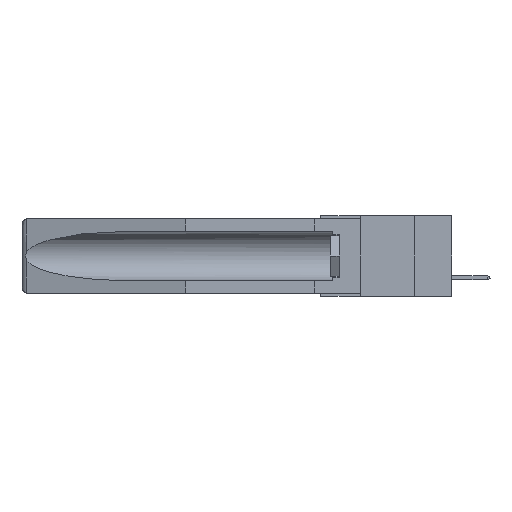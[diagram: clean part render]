
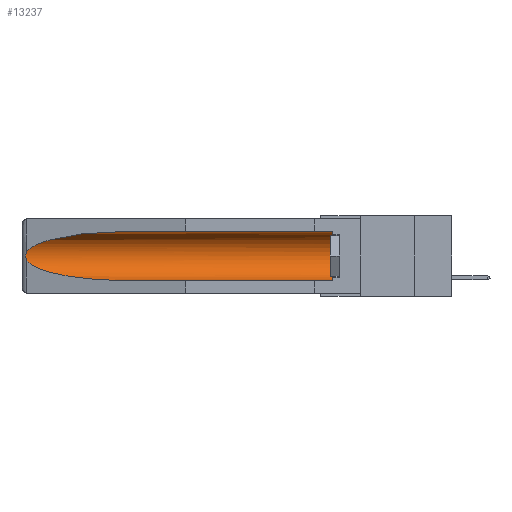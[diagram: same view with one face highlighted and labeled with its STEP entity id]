
A CAD part, left-side view. The second image highlights one B-rep face of the part: STEP entity #13237.
In plain terms, the highlighted cylindrical face has radius 2.857 mm (diameter 5.715 mm), a partial arc.
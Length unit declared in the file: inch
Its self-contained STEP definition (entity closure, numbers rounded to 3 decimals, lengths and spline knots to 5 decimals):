
#164 = CARTESIAN_POINT ( 'NONE',  ( 0.25451, 1.48313, -0.24835 ) ) ;
#382 = CARTESIAN_POINT ( 'NONE',  ( 0.25451, 1.48313, -0.09465 ) ) ;
#494 = CARTESIAN_POINT ( 'NONE',  ( 0.26537, 1.52718, -0.14972 ) ) ;
#1466 = CARTESIAN_POINT ( 'NONE',  ( 0.155, -0.30754, -0.1715 ) ) ;
#1634 = ORIENTED_EDGE ( 'NONE', *, *, #14300, .T. ) ;
#1669 = CARTESIAN_POINT ( 'NONE',  ( 0.2675, 1.53308, -0.16763 ) ) ;
#1854 = CARTESIAN_POINT ( 'NONE',  ( 0.155, -0.30754, -0.059 ) ) ;
#1901 = EDGE_CURVE ( 'NONE', #17333, #27058, #24719, .T. ) ;
#3389 = CARTESIAN_POINT ( 'NONE',  ( 0.155, 0.126, -0.1715 ) ) ;
#4767 = AXIS2_PLACEMENT_3D ( 'NONE', #1466, #8521, #29574 ) ;
#5456 = EDGE_LOOP ( 'NONE', ( #8211, #10354, #6755, #15184, #1634, #26375 ) ) ;
#6057 = CARTESIAN_POINT ( 'NONE',  ( 0.26537, 1.52718, -0.14972 ) ) ;
#6107 = CARTESIAN_POINT ( 'NONE',  ( 0.26655, 1.53094, -0.18657 ) ) ;
#6202 = CARTESIAN_POINT ( 'NONE',  ( 0.26537, 1.52718, -0.19328 ) ) ;
#6246 = CARTESIAN_POINT ( 'NONE',  ( 0.155, 0.126, -0.059 ) ) ;
#6336 = VERTEX_POINT ( 'NONE', #13938 ) ;
#6755 = ORIENTED_EDGE ( 'NONE', *, *, #1901, .T. ) ;
#8211 = ORIENTED_EDGE ( 'NONE', *, *, #19266, .T. ) ;
#8521 = DIRECTION ( 'NONE',  ( 0., 1., 0. ) ) ;
#8726 = CARTESIAN_POINT ( 'NONE',  ( 0.26597, 1.52961, -0.15275 ) ) ;
#9156 = VERTEX_POINT ( 'NONE', #6057 ) ;
#9157 = LINE ( 'NONE', #1854, #20053 ) ;
#10107 = VERTEX_POINT ( 'NONE', #29409 ) ;
#10354 = ORIENTED_EDGE ( 'NONE', *, *, #13172, .T. ) ;
#10546 = DIRECTION ( 'NONE',  ( 0., 0., 1. ) ) ;
#10957 = CARTESIAN_POINT ( 'NONE',  ( 0.26537, 1.52718, -0.14972 ) ) ;
#11057 = CARTESIAN_POINT ( 'NONE',  ( 0.26597, 1.5296, -0.19026 ) ) ;
#11389 = EDGE_CURVE ( 'NONE', #10107, #27058, #13579, .T. ) ;
#11465 = FACE_OUTER_BOUND ( 'NONE', #5456, .T. ) ;
#11480 = DIRECTION ( 'NONE',  ( 0., 1., 0. ) ) ;
#12417 = DIRECTION ( 'NONE',  ( 0., 1., 0. ) ) ;
#13117 = CARTESIAN_POINT ( 'NONE',  ( 0.2673, 1.53269, -0.17917 ) ) ;
#13172 = EDGE_CURVE ( 'NONE', #9156, #17333, #25464, .T. ) ;
#13237 = ADVANCED_FACE ( 'NONE', ( #11465 ), #24193, .F. ) ;
#13579 = LINE ( 'NONE', #26346, #15767 ) ;
#13938 = CARTESIAN_POINT ( 'NONE',  ( 0.155, 1.07973, -0.059 ) ) ;
#14228 = CARTESIAN_POINT ( 'NONE',  ( 0.26537, 1.52718, -0.19328 ) ) ;
#14300 = EDGE_CURVE ( 'NONE', #10107, #16545, #23719, .T. ) ;
#14334 = CARTESIAN_POINT ( 'NONE',  ( 0.155, 1.07973, -0.284 ) ) ;
#15184 = ORIENTED_EDGE ( 'NONE', *, *, #11389, .F. ) ;
#15767 = VECTOR ( 'NONE', #12417, 39.37008 ) ;
#16545 = VERTEX_POINT ( 'NONE', #6246 ) ;
#17333 = VERTEX_POINT ( 'NONE', #28161 ) ;
#17841 = CARTESIAN_POINT ( 'NONE',  ( 0.2675, 1.53308, -0.17534 ) ) ;
#18059 = CARTESIAN_POINT ( 'NONE',  ( 0.2673, 1.5327, -0.16383 ) ) ;
#18617 = CARTESIAN_POINT ( 'NONE',  ( 0.21114, 1.30732, -0.059 ) ) ;
#18692 = CARTESIAN_POINT ( 'NONE',  ( 0.21114, 1.30732, -0.284 ) ) ;
#19266 = EDGE_CURVE ( 'NONE', #6336, #9156, #21499, .T. ) ;
#20053 = VECTOR ( 'NONE', #11480, 39.37008 ) ;
#20188 = AXIS2_PLACEMENT_3D ( 'NONE', #3389, #26691, #10546 ) ;
#21499 =( BOUNDED_CURVE ( )  B_SPLINE_CURVE ( 3, ( #28031, #18617, #382, #494 ),
 .UNSPECIFIED., .F., .F. ) 
 B_SPLINE_CURVE_WITH_KNOTS ( ( 4, 4 ),
 ( 4.71239, 6.08839 ),
 .UNSPECIFIED. ) 
 CURVE ( )  GEOMETRIC_REPRESENTATION_ITEM ( )  RATIONAL_B_SPLINE_CURVE ( ( 1., 0.848, 0.848, 1. ) ) 
 REPRESENTATION_ITEM ( '' )  );
#21911 = EDGE_CURVE ( 'NONE', #16545, #6336, #9157, .T. ) ;
#22880 = CARTESIAN_POINT ( 'NONE',  ( 0.155, 1.07973, -0.284 ) ) ;
#23719 = CIRCLE ( 'NONE', #20188, 0.1125 ) ;
#24193 = CYLINDRICAL_SURFACE ( 'NONE', #4767, 0.1125 ) ;
#24719 =( BOUNDED_CURVE ( )  B_SPLINE_CURVE ( 3, ( #14228, #164, #18692, #14334 ),
 .UNSPECIFIED., .F., .F. ) 
 B_SPLINE_CURVE_WITH_KNOTS ( ( 4, 4 ),
 ( 0.1948, 1.5708 ),
 .UNSPECIFIED. ) 
 CURVE ( )  GEOMETRIC_REPRESENTATION_ITEM ( )  RATIONAL_B_SPLINE_CURVE ( ( 1., 0.848, 0.848, 1. ) ) 
 REPRESENTATION_ITEM ( '' )  );
#25464 = B_SPLINE_CURVE_WITH_KNOTS ( 'NONE', 3,
 ( #10957, #8726, #27130, #18059, #1669, #17841, #13117, #6107, #11057, #6202 ),
 .UNSPECIFIED., .F., .F.,
 ( 4, 2, 2, 2, 4 ),
 ( 0., 0.00029, 0.00058, 0.00087, 0.00117 ),
 .UNSPECIFIED. ) ;
#26346 = CARTESIAN_POINT ( 'NONE',  ( 0.155, -0.30754, -0.284 ) ) ;
#26375 = ORIENTED_EDGE ( 'NONE', *, *, #21911, .T. ) ;
#26691 = DIRECTION ( 'NONE',  ( 0., -1., 0. ) ) ;
#27058 = VERTEX_POINT ( 'NONE', #22880 ) ;
#27130 = CARTESIAN_POINT ( 'NONE',  ( 0.26654, 1.53092, -0.15636 ) ) ;
#28031 = CARTESIAN_POINT ( 'NONE',  ( 0.155, 1.07973, -0.059 ) ) ;
#28161 = CARTESIAN_POINT ( 'NONE',  ( 0.26537, 1.52718, -0.19328 ) ) ;
#29409 = CARTESIAN_POINT ( 'NONE',  ( 0.155, 0.126, -0.284 ) ) ;
#29574 = DIRECTION ( 'NONE',  ( 0., 0., 1. ) ) ;
